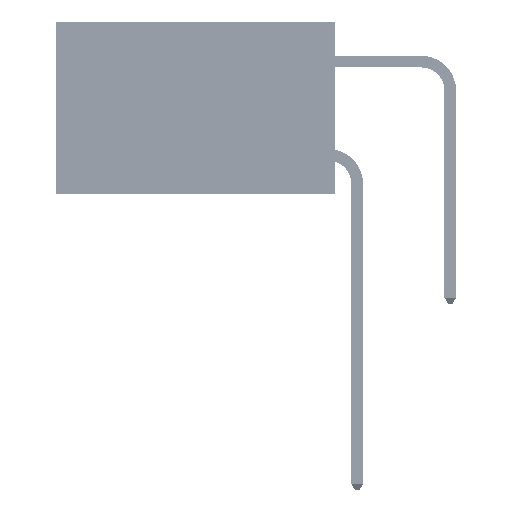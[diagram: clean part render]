
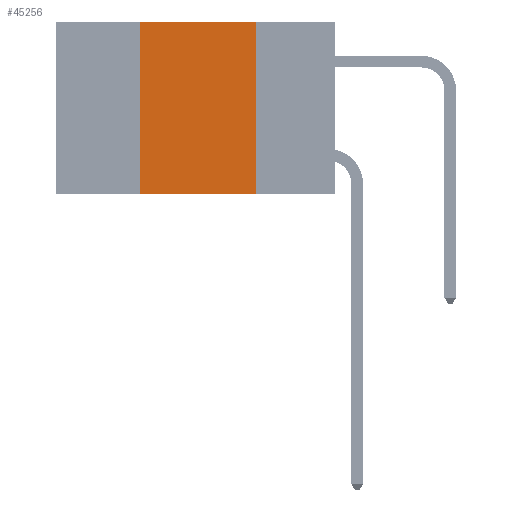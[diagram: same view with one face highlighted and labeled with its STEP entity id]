
A CAD part, left-side view. The second image highlights one B-rep face of the part: STEP entity #45256.
In plain terms, the highlighted planar face has unit normal (-1, 0, 0).
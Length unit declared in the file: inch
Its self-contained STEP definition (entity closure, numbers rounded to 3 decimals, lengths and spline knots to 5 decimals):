
#159 = LINE ( 'NONE', #40360, #41136 ) ;
#1184 = VECTOR ( 'NONE', #26367, 39.37008 ) ;
#1882 = CARTESIAN_POINT ( 'NONE',  ( 0., 0.42, -0.37 ) ) ;
#4152 = VECTOR ( 'NONE', #4529, 39.37008 ) ;
#4529 = DIRECTION ( 'NONE',  ( 0., 0., -1. ) ) ;
#5088 = VERTEX_POINT ( 'NONE', #1882 ) ;
#5283 = DIRECTION ( 'NONE',  ( 1., 0., 0. ) ) ;
#5740 = FACE_OUTER_BOUND ( 'NONE', #20330, .T. ) ;
#6036 = AXIS2_PLACEMENT_3D ( 'NONE', #38243, #5283, #42097 ) ;
#7875 = EDGE_CURVE ( 'NONE', #5088, #29068, #14408, .T. ) ;
#9618 = ORIENTED_EDGE ( 'NONE', *, *, #26890, .T. ) ;
#10904 = VERTEX_POINT ( 'NONE', #20295 ) ;
#14408 = LINE ( 'NONE', #18003, #38516 ) ;
#16344 = CARTESIAN_POINT ( 'NONE',  ( 0., 0.17, 0. ) ) ;
#16368 = CARTESIAN_POINT ( 'NONE',  ( 0., 0.42, 0. ) ) ;
#18003 = CARTESIAN_POINT ( 'NONE',  ( 0., 0.42, 0. ) ) ;
#20295 = CARTESIAN_POINT ( 'NONE',  ( 0., 0.17, -0.37 ) ) ;
#20330 = EDGE_LOOP ( 'NONE', ( #25431, #22255, #41454, #9618 ) ) ;
#21382 = DIRECTION ( 'NONE',  ( 0., 0., 1. ) ) ;
#22255 = ORIENTED_EDGE ( 'NONE', *, *, #40217, .F. ) ;
#23553 = PLANE ( 'NONE',  #6036 ) ;
#25431 = ORIENTED_EDGE ( 'NONE', *, *, #38461, .F. ) ;
#26367 = DIRECTION ( 'NONE',  ( 0., -1., 0. ) ) ;
#26890 = EDGE_CURVE ( 'NONE', #5088, #10904, #159, .T. ) ;
#26895 = LINE ( 'NONE', #41106, #4152 ) ;
#29068 = VERTEX_POINT ( 'NONE', #16368 ) ;
#36760 = DIRECTION ( 'NONE',  ( 0., -1., 0. ) ) ;
#37681 = LINE ( 'NONE', #44668, #1184 ) ;
#38243 = CARTESIAN_POINT ( 'NONE',  ( 0., 0.6, 0. ) ) ;
#38461 = EDGE_CURVE ( 'NONE', #41942, #10904, #26895, .T. ) ;
#38516 = VECTOR ( 'NONE', #21382, 39.37008 ) ;
#40217 = EDGE_CURVE ( 'NONE', #29068, #41942, #37681, .T. ) ;
#40360 = CARTESIAN_POINT ( 'NONE',  ( 0., 0.6, -0.37 ) ) ;
#41106 = CARTESIAN_POINT ( 'NONE',  ( 0., 0.17, 0. ) ) ;
#41136 = VECTOR ( 'NONE', #36760, 39.37008 ) ;
#41454 = ORIENTED_EDGE ( 'NONE', *, *, #7875, .F. ) ;
#41942 = VERTEX_POINT ( 'NONE', #16344 ) ;
#42097 = DIRECTION ( 'NONE',  ( 0., 0., -1. ) ) ;
#44668 = CARTESIAN_POINT ( 'NONE',  ( 0., 0.6, 0. ) ) ;
#45256 = ADVANCED_FACE ( 'NONE', ( #5740 ), #23553, .F. ) ;
